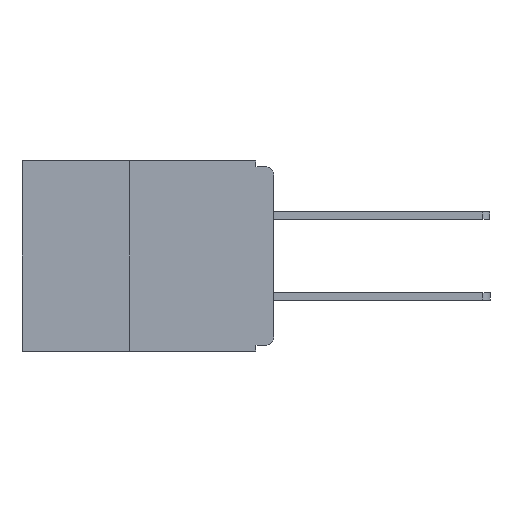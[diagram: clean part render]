
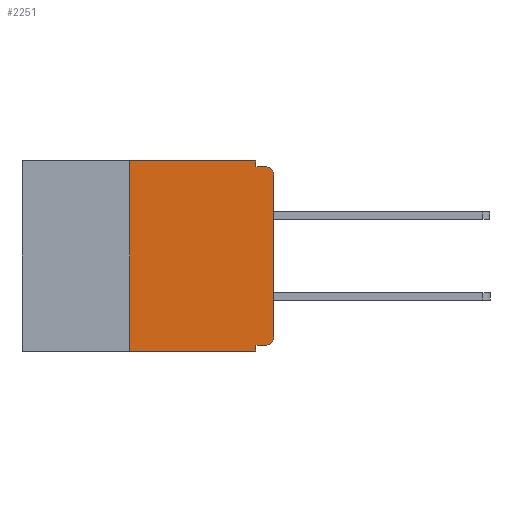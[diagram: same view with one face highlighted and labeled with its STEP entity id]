
A CAD part, left-side view. The second image highlights one B-rep face of the part: STEP entity #2251.
In plain terms, the highlighted planar face has unit normal (-1, 0, 0).
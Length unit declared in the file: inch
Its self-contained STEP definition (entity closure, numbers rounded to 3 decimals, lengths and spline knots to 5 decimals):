
#53 = ORIENTED_EDGE ( 'NONE', *, *, #10990, .F. ) ;
#398 = LINE ( 'NONE', #11091, #3475 ) ;
#504 = CARTESIAN_POINT ( 'NONE',  ( 0., 0., -0.305 ) ) ;
#684 = VERTEX_POINT ( 'NONE', #13166 ) ;
#784 = LINE ( 'NONE', #16455, #15604 ) ;
#838 = EDGE_CURVE ( 'NONE', #16955, #4098, #2503, .T. ) ;
#860 = DIRECTION ( 'NONE',  ( 0., 0., 1. ) ) ;
#1418 = ORIENTED_EDGE ( 'NONE', *, *, #1476, .T. ) ;
#1476 = EDGE_CURVE ( 'NONE', #12098, #11563, #4182, .T. ) ;
#1826 = CARTESIAN_POINT ( 'NONE',  ( 0., 0., -0.32 ) ) ;
#1959 = LINE ( 'NONE', #2107, #6325 ) ;
#1979 = AXIS2_PLACEMENT_3D ( 'NONE', #5135, #5145, #2266 ) ;
#2007 = AXIS2_PLACEMENT_3D ( 'NONE', #13353, #7296, #14150 ) ;
#2107 = CARTESIAN_POINT ( 'NONE',  ( 0., 0.437, 0. ) ) ;
#2251 = ADVANCED_FACE ( 'NONE', ( #15207 ), #9082, .F. ) ;
#2266 = DIRECTION ( 'NONE',  ( 0., 0., -1. ) ) ;
#2498 = EDGE_CURVE ( 'NONE', #3528, #10826, #784, .T. ) ;
#2503 = LINE ( 'NONE', #5845, #6394 ) ;
#3475 = VECTOR ( 'NONE', #12457, 39.37008 ) ;
#3528 = VERTEX_POINT ( 'NONE', #8469 ) ;
#3633 = ORIENTED_EDGE ( 'NONE', *, *, #4053, .F. ) ;
#4053 = EDGE_CURVE ( 'NONE', #10826, #11563, #15356, .T. ) ;
#4098 = VERTEX_POINT ( 'NONE', #8918 ) ;
#4182 = CIRCLE ( 'NONE', #1979, 0.015 ) ;
#4184 = LINE ( 'NONE', #14673, #14631 ) ;
#4539 = VERTEX_POINT ( 'NONE', #6227 ) ;
#4884 = EDGE_CURVE ( 'NONE', #12327, #8753, #8011, .T. ) ;
#5135 = CARTESIAN_POINT ( 'NONE',  ( 0., 0.015, -0.025 ) ) ;
#5145 = DIRECTION ( 'NONE',  ( -1., 0., 0. ) ) ;
#5375 = EDGE_CURVE ( 'NONE', #12327, #4539, #14701, .T. ) ;
#5565 = AXIS2_PLACEMENT_3D ( 'NONE', #8159, #17384, #9535 ) ;
#5595 = ORIENTED_EDGE ( 'NONE', *, *, #16049, .T. ) ;
#5597 = DIRECTION ( 'NONE',  ( 0., 0., 1. ) ) ;
#5845 = CARTESIAN_POINT ( 'NONE',  ( 0., 0.25, -0.33 ) ) ;
#6078 = ORIENTED_EDGE ( 'NONE', *, *, #838, .F. ) ;
#6227 = CARTESIAN_POINT ( 'NONE',  ( 0., 0.031, -0.32 ) ) ;
#6325 = VECTOR ( 'NONE', #12014, 39.37008 ) ;
#6394 = VECTOR ( 'NONE', #5597, 39.37008 ) ;
#6740 = CARTESIAN_POINT ( 'NONE',  ( 0., 0., 0. ) ) ;
#7296 = DIRECTION ( 'NONE',  ( 1., 0., 0. ) ) ;
#8011 = CIRCLE ( 'NONE', #5565, 0.015 ) ;
#8017 = ORIENTED_EDGE ( 'NONE', *, *, #8068, .T. ) ;
#8032 = ORIENTED_EDGE ( 'NONE', *, *, #15224, .F. ) ;
#8068 = EDGE_CURVE ( 'NONE', #8753, #12098, #14622, .T. ) ;
#8159 = CARTESIAN_POINT ( 'NONE',  ( 0., 0.015, -0.305 ) ) ;
#8204 = EDGE_LOOP ( 'NONE', ( #8017, #1418, #3633, #15030, #53, #6078, #5595, #8032, #12714, #13477 ) ) ;
#8469 = CARTESIAN_POINT ( 'NONE',  ( 0., 0.031, 0. ) ) ;
#8753 = VERTEX_POINT ( 'NONE', #504 ) ;
#8918 = CARTESIAN_POINT ( 'NONE',  ( 0., 0.25, 0. ) ) ;
#9082 = PLANE ( 'NONE',  #2007 ) ;
#9535 = DIRECTION ( 'NONE',  ( 0., 0., -1. ) ) ;
#10826 = VERTEX_POINT ( 'NONE', #12912 ) ;
#10961 = CARTESIAN_POINT ( 'NONE',  ( 0., 0., -0.025 ) ) ;
#10990 = EDGE_CURVE ( 'NONE', #4098, #3528, #1959, .T. ) ;
#11091 = CARTESIAN_POINT ( 'NONE',  ( 0., 0.437, -0.33 ) ) ;
#11220 = VECTOR ( 'NONE', #16928, 39.37008 ) ;
#11365 = DIRECTION ( 'NONE',  ( 0., -1., 0. ) ) ;
#11519 = CARTESIAN_POINT ( 'NONE',  ( 0., 0., -0.01 ) ) ;
#11563 = VERTEX_POINT ( 'NONE', #11656 ) ;
#11656 = CARTESIAN_POINT ( 'NONE',  ( 0., 0.015, -0.01 ) ) ;
#11900 = VECTOR ( 'NONE', #11365, 39.37008 ) ;
#12014 = DIRECTION ( 'NONE',  ( 0., -1., 0. ) ) ;
#12098 = VERTEX_POINT ( 'NONE', #10961 ) ;
#12327 = VERTEX_POINT ( 'NONE', #16584 ) ;
#12457 = DIRECTION ( 'NONE',  ( 0., -1., 0. ) ) ;
#12714 = ORIENTED_EDGE ( 'NONE', *, *, #5375, .F. ) ;
#12912 = CARTESIAN_POINT ( 'NONE',  ( 0., 0.031, -0.01 ) ) ;
#13166 = CARTESIAN_POINT ( 'NONE',  ( 0., 0.031, -0.33 ) ) ;
#13353 = CARTESIAN_POINT ( 'NONE',  ( 0., 0.437, 0. ) ) ;
#13477 = ORIENTED_EDGE ( 'NONE', *, *, #4884, .T. ) ;
#14150 = DIRECTION ( 'NONE',  ( 0., 0., -1. ) ) ;
#14622 = LINE ( 'NONE', #6740, #17608 ) ;
#14631 = VECTOR ( 'NONE', #15949, 39.37008 ) ;
#14673 = CARTESIAN_POINT ( 'NONE',  ( 0., 0.031, -0.33 ) ) ;
#14701 = LINE ( 'NONE', #1826, #11220 ) ;
#15030 = ORIENTED_EDGE ( 'NONE', *, *, #2498, .F. ) ;
#15207 = FACE_OUTER_BOUND ( 'NONE', #8204, .T. ) ;
#15224 = EDGE_CURVE ( 'NONE', #4539, #684, #4184, .T. ) ;
#15266 = CARTESIAN_POINT ( 'NONE',  ( 0., 0.25, -0.33 ) ) ;
#15356 = LINE ( 'NONE', #11519, #11900 ) ;
#15604 = VECTOR ( 'NONE', #16361, 39.37008 ) ;
#15949 = DIRECTION ( 'NONE',  ( 0., 0., -1. ) ) ;
#16049 = EDGE_CURVE ( 'NONE', #16955, #684, #398, .T. ) ;
#16361 = DIRECTION ( 'NONE',  ( 0., 0., -1. ) ) ;
#16455 = CARTESIAN_POINT ( 'NONE',  ( 0., 0.031, 0. ) ) ;
#16584 = CARTESIAN_POINT ( 'NONE',  ( 0., 0.015, -0.32 ) ) ;
#16928 = DIRECTION ( 'NONE',  ( 0., 1., 0. ) ) ;
#16955 = VERTEX_POINT ( 'NONE', #15266 ) ;
#17384 = DIRECTION ( 'NONE',  ( -1., 0., 0. ) ) ;
#17608 = VECTOR ( 'NONE', #860, 39.37008 ) ;
